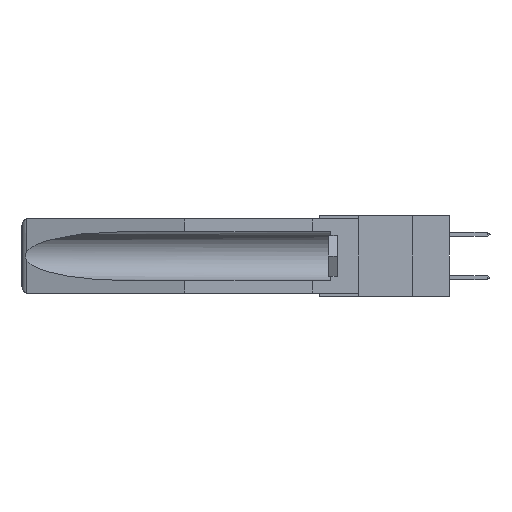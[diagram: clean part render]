
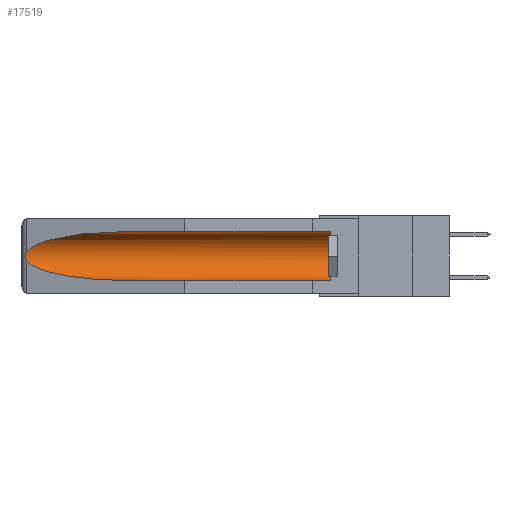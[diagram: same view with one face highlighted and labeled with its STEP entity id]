
A CAD part, left-side view. The second image highlights one B-rep face of the part: STEP entity #17519.
In plain terms, the highlighted cylindrical face has radius 2.857 mm (diameter 5.715 mm), a partial arc.
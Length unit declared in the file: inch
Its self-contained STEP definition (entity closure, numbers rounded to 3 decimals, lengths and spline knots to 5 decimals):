
#646 = CARTESIAN_POINT ( 'NONE',  ( 0.155, -0.30754, -0.284 ) ) ;
#1258 = CARTESIAN_POINT ( 'NONE',  ( 0.26537, 1.52718, -0.19328 ) ) ;
#1830 = VERTEX_POINT ( 'NONE', #12738 ) ;
#2304 = CARTESIAN_POINT ( 'NONE',  ( 0.25451, 1.48313, -0.24835 ) ) ;
#2446 = CARTESIAN_POINT ( 'NONE',  ( 0.21114, 1.30732, -0.284 ) ) ;
#2673 = LINE ( 'NONE', #646, #20218 ) ;
#3387 = AXIS2_PLACEMENT_3D ( 'NONE', #21052, #6332, #12874 ) ;
#4619 = EDGE_LOOP ( 'NONE', ( #13407, #15932, #15042, #5207, #18445, #13164 ) ) ;
#5207 = ORIENTED_EDGE ( 'NONE', *, *, #15673, .F. ) ;
#5487 = CARTESIAN_POINT ( 'NONE',  ( 0.155, -0.30754, -0.059 ) ) ;
#6332 = DIRECTION ( 'NONE',  ( 0., 1., 0. ) ) ;
#6368 = VERTEX_POINT ( 'NONE', #7376 ) ;
#6589 = VERTEX_POINT ( 'NONE', #15770 ) ;
#7376 = CARTESIAN_POINT ( 'NONE',  ( 0.26537, 1.52718, -0.14972 ) ) ;
#7749 = DIRECTION ( 'NONE',  ( 0., -1., 0. ) ) ;
#8617 = CARTESIAN_POINT ( 'NONE',  ( 0.155, 1.07973, -0.059 ) ) ;
#9991 = EDGE_CURVE ( 'NONE', #16858, #6368, #10925, .T. ) ;
#10173 = CARTESIAN_POINT ( 'NONE',  ( 0.21114, 1.30732, -0.059 ) ) ;
#10416 = EDGE_CURVE ( 'NONE', #20746, #6589, #20188, .T. ) ;
#10705 = CARTESIAN_POINT ( 'NONE',  ( 0.26597, 1.52961, -0.15275 ) ) ;
#10841 = CARTESIAN_POINT ( 'NONE',  ( 0.26655, 1.53094, -0.18657 ) ) ;
#10857 = LINE ( 'NONE', #5487, #18495 ) ;
#10925 =( BOUNDED_CURVE ( )  B_SPLINE_CURVE ( 3, ( #8617, #10173, #16800, #20216 ),
 .UNSPECIFIED., .F., .F. ) 
 B_SPLINE_CURVE_WITH_KNOTS ( ( 4, 4 ),
 ( 4.71239, 6.08839 ),
 .UNSPECIFIED. ) 
 CURVE ( )  GEOMETRIC_REPRESENTATION_ITEM ( )  RATIONAL_B_SPLINE_CURVE ( ( 1., 0.848, 0.848, 1. ) ) 
 REPRESENTATION_ITEM ( '' )  );
#11688 = B_SPLINE_CURVE_WITH_KNOTS ( 'NONE', 3,
 ( #20341, #10705, #18955, #12701, #15890, #17586, #12553, #10841, #15769, #1258 ),
 .UNSPECIFIED., .F., .F.,
 ( 4, 2, 2, 2, 4 ),
 ( 0., 0.00029, 0.00058, 0.00087, 0.00117 ),
 .UNSPECIFIED. ) ;
#12020 = CARTESIAN_POINT ( 'NONE',  ( 0.26537, 1.52718, -0.19328 ) ) ;
#12124 = VERTEX_POINT ( 'NONE', #20385 ) ;
#12553 = CARTESIAN_POINT ( 'NONE',  ( 0.2673, 1.53269, -0.17917 ) ) ;
#12701 = CARTESIAN_POINT ( 'NONE',  ( 0.2673, 1.5327, -0.16383 ) ) ;
#12738 = CARTESIAN_POINT ( 'NONE',  ( 0.26537, 1.52718, -0.19328 ) ) ;
#12739 = CARTESIAN_POINT ( 'NONE',  ( 0.155, 0.126, -0.1715 ) ) ;
#12874 = DIRECTION ( 'NONE',  ( 0., 0., 1. ) ) ;
#12904 = CARTESIAN_POINT ( 'NONE',  ( 0.155, 1.07973, -0.059 ) ) ;
#13164 = ORIENTED_EDGE ( 'NONE', *, *, #17160, .T. ) ;
#13407 = ORIENTED_EDGE ( 'NONE', *, *, #9991, .T. ) ;
#13527 = CARTESIAN_POINT ( 'NONE',  ( 0.155, 0.126, -0.284 ) ) ;
#15042 = ORIENTED_EDGE ( 'NONE', *, *, #15526, .T. ) ;
#15077 = DIRECTION ( 'NONE',  ( 0., 1., 0. ) ) ;
#15091 =( BOUNDED_CURVE ( )  B_SPLINE_CURVE ( 3, ( #12020, #2304, #2446, #16942 ),
 .UNSPECIFIED., .F., .F. ) 
 B_SPLINE_CURVE_WITH_KNOTS ( ( 4, 4 ),
 ( 0.1948, 1.5708 ),
 .UNSPECIFIED. ) 
 CURVE ( )  GEOMETRIC_REPRESENTATION_ITEM ( )  RATIONAL_B_SPLINE_CURVE ( ( 1., 0.848, 0.848, 1. ) ) 
 REPRESENTATION_ITEM ( '' )  );
#15526 = EDGE_CURVE ( 'NONE', #1830, #12124, #15091, .T. ) ;
#15673 = EDGE_CURVE ( 'NONE', #20746, #12124, #2673, .T. ) ;
#15770 = CARTESIAN_POINT ( 'NONE',  ( 0.155, 0.126, -0.059 ) ) ;
#15769 = CARTESIAN_POINT ( 'NONE',  ( 0.26597, 1.5296, -0.19026 ) ) ;
#15890 = CARTESIAN_POINT ( 'NONE',  ( 0.2675, 1.53308, -0.16763 ) ) ;
#15932 = ORIENTED_EDGE ( 'NONE', *, *, #18621, .T. ) ;
#16669 = DIRECTION ( 'NONE',  ( 0., 1., 0. ) ) ;
#16800 = CARTESIAN_POINT ( 'NONE',  ( 0.25451, 1.48313, -0.09465 ) ) ;
#16858 = VERTEX_POINT ( 'NONE', #12904 ) ;
#16942 = CARTESIAN_POINT ( 'NONE',  ( 0.155, 1.07973, -0.284 ) ) ;
#17160 = EDGE_CURVE ( 'NONE', #6589, #16858, #10857, .T. ) ;
#17519 = ADVANCED_FACE ( 'NONE', ( #20529 ), #20018, .F. ) ;
#17586 = CARTESIAN_POINT ( 'NONE',  ( 0.2675, 1.53308, -0.17534 ) ) ;
#18445 = ORIENTED_EDGE ( 'NONE', *, *, #10416, .T. ) ;
#18495 = VECTOR ( 'NONE', #16669, 39.37008 ) ;
#18621 = EDGE_CURVE ( 'NONE', #6368, #1830, #11688, .T. ) ;
#18955 = CARTESIAN_POINT ( 'NONE',  ( 0.26654, 1.53092, -0.15636 ) ) ;
#19276 = DIRECTION ( 'NONE',  ( 0., 0., 1. ) ) ;
#20018 = CYLINDRICAL_SURFACE ( 'NONE', #3387, 0.1125 ) ;
#20188 = CIRCLE ( 'NONE', #21078, 0.1125 ) ;
#20216 = CARTESIAN_POINT ( 'NONE',  ( 0.26537, 1.52718, -0.14972 ) ) ;
#20218 = VECTOR ( 'NONE', #15077, 39.37008 ) ;
#20341 = CARTESIAN_POINT ( 'NONE',  ( 0.26537, 1.52718, -0.14972 ) ) ;
#20385 = CARTESIAN_POINT ( 'NONE',  ( 0.155, 1.07973, -0.284 ) ) ;
#20529 = FACE_OUTER_BOUND ( 'NONE', #4619, .T. ) ;
#20746 = VERTEX_POINT ( 'NONE', #13527 ) ;
#21052 = CARTESIAN_POINT ( 'NONE',  ( 0.155, -0.30754, -0.1715 ) ) ;
#21078 = AXIS2_PLACEMENT_3D ( 'NONE', #12739, #7749, #19276 ) ;
